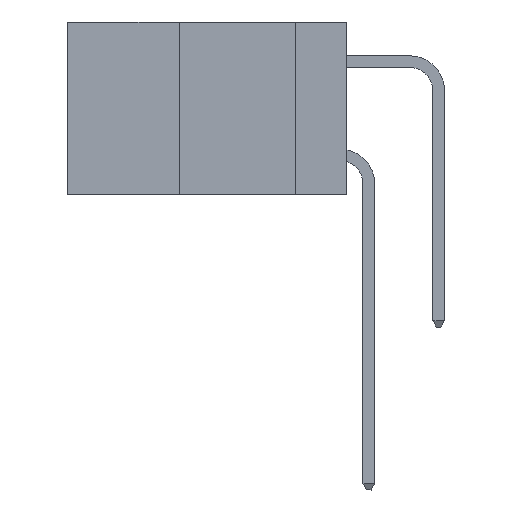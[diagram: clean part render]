
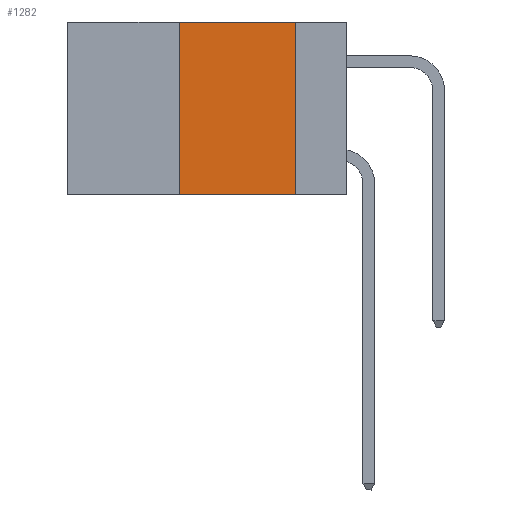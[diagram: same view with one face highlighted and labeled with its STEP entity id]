
A CAD part, left-side view. The second image highlights one B-rep face of the part: STEP entity #1282.
In plain terms, the highlighted planar face has unit normal (-1, 0, 0).
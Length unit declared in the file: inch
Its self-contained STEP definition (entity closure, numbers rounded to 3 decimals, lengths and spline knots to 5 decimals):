
#319 = CARTESIAN_POINT ( 'NONE',  ( 0., 0.36, 0. ) ) ;
#636 = EDGE_CURVE ( 'NONE', #9484, #894, #2992, .T. ) ;
#652 = CARTESIAN_POINT ( 'NONE',  ( 0., 0.11, 0. ) ) ;
#894 = VERTEX_POINT ( 'NONE', #2611 ) ;
#961 = ORIENTED_EDGE ( 'NONE', *, *, #18060, .T. ) ;
#1206 = EDGE_CURVE ( 'NONE', #13176, #9484, #20879, .T. ) ;
#1282 = ADVANCED_FACE ( 'NONE', ( #12597 ), #11344, .F. ) ;
#1798 = DIRECTION ( 'NONE',  ( 0., -1., 0. ) ) ;
#1890 = EDGE_LOOP ( 'NONE', ( #13213, #15040, #11507, #961 ) ) ;
#1947 = VECTOR ( 'NONE', #5206, 39.37008 ) ;
#2611 = CARTESIAN_POINT ( 'NONE',  ( 0., 0.11, -0.37 ) ) ;
#2809 = DIRECTION ( 'NONE',  ( 0., 0., -1. ) ) ;
#2887 = DIRECTION ( 'NONE',  ( 0., 0., -1. ) ) ;
#2992 = LINE ( 'NONE', #10066, #4996 ) ;
#3936 = CARTESIAN_POINT ( 'NONE',  ( 0., 0.6, 0. ) ) ;
#4390 = DIRECTION ( 'NONE',  ( 1., 0., 0. ) ) ;
#4996 = VECTOR ( 'NONE', #2887, 39.37008 ) ;
#5206 = DIRECTION ( 'NONE',  ( 0., 0., 1. ) ) ;
#6180 = CARTESIAN_POINT ( 'NONE',  ( 0., 0.6, 0. ) ) ;
#6627 = LINE ( 'NONE', #6966, #7828 ) ;
#6966 = CARTESIAN_POINT ( 'NONE',  ( 0., 0.6, -0.37 ) ) ;
#7515 = VERTEX_POINT ( 'NONE', #10854 ) ;
#7828 = VECTOR ( 'NONE', #1798, 39.37008 ) ;
#9484 = VERTEX_POINT ( 'NONE', #652 ) ;
#10066 = CARTESIAN_POINT ( 'NONE',  ( 0., 0.11, 0. ) ) ;
#10854 = CARTESIAN_POINT ( 'NONE',  ( 0., 0.36, -0.37 ) ) ;
#11344 = PLANE ( 'NONE',  #17928 ) ;
#11507 = ORIENTED_EDGE ( 'NONE', *, *, #11861, .F. ) ;
#11861 = EDGE_CURVE ( 'NONE', #7515, #13176, #15531, .T. ) ;
#12554 = VECTOR ( 'NONE', #15628, 39.37008 ) ;
#12597 = FACE_OUTER_BOUND ( 'NONE', #1890, .T. ) ;
#13176 = VERTEX_POINT ( 'NONE', #319 ) ;
#13213 = ORIENTED_EDGE ( 'NONE', *, *, #636, .F. ) ;
#13962 = CARTESIAN_POINT ( 'NONE',  ( 0., 0.36, 0. ) ) ;
#15040 = ORIENTED_EDGE ( 'NONE', *, *, #1206, .F. ) ;
#15531 = LINE ( 'NONE', #13962, #1947 ) ;
#15628 = DIRECTION ( 'NONE',  ( 0., -1., 0. ) ) ;
#17928 = AXIS2_PLACEMENT_3D ( 'NONE', #6180, #4390, #2809 ) ;
#18060 = EDGE_CURVE ( 'NONE', #7515, #894, #6627, .T. ) ;
#20879 = LINE ( 'NONE', #3936, #12554 ) ;
